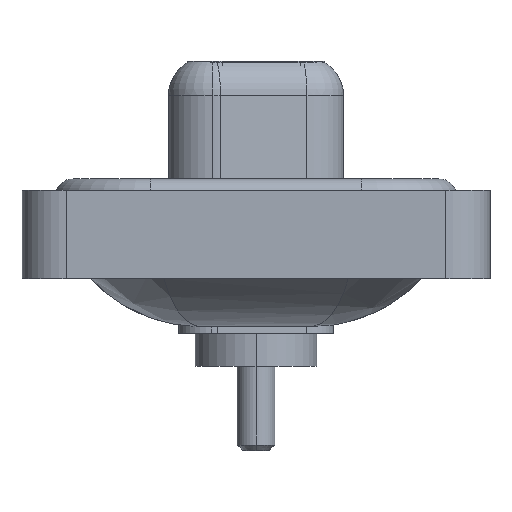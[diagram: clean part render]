
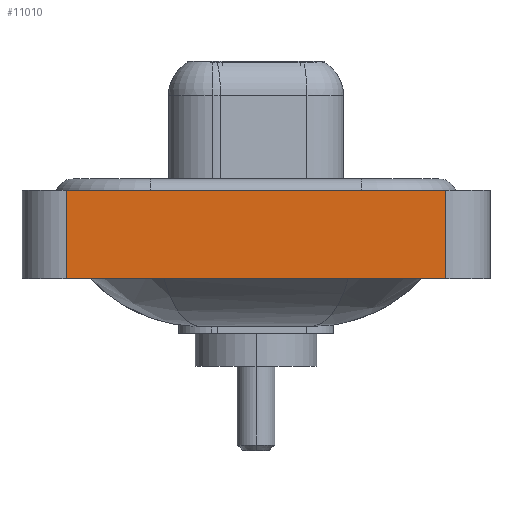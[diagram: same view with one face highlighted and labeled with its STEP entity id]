
A CAD part, left-side view. The second image highlights one B-rep face of the part: STEP entity #11010.
In plain terms, the highlighted planar face has unit normal (-1, 0, 0).
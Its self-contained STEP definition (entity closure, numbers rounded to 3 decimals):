
#503 = VERTEX_POINT ( 'NONE', #1447 ) ;
#768 = CARTESIAN_POINT ( 'NONE',  ( -7.25, 8.55, -3.6 ) ) ;
#1003 = VECTOR ( 'NONE', #8576, 1000. ) ;
#1018 = FACE_OUTER_BOUND ( 'NONE', #13302, .T. ) ;
#1052 = ORIENTED_EDGE ( 'NONE', *, *, #15396, .T. ) ;
#1237 = VECTOR ( 'NONE', #14821, 1000. ) ;
#1447 = CARTESIAN_POINT ( 'NONE',  ( -7.25, -8.55, 0.4 ) ) ;
#2682 = DIRECTION ( 'NONE',  ( -1., 0., 0. ) ) ;
#2829 = CARTESIAN_POINT ( 'NONE',  ( -7.25, -8.55, -3.6 ) ) ;
#3070 = CARTESIAN_POINT ( 'NONE',  ( -7.25, -8.55, 0.4 ) ) ;
#3627 = PLANE ( 'NONE',  #10861 ) ;
#4041 = VECTOR ( 'NONE', #7877, 1000. ) ;
#4417 = LINE ( 'NONE', #3070, #8654 ) ;
#5239 = VERTEX_POINT ( 'NONE', #16526 ) ;
#5352 = CARTESIAN_POINT ( 'NONE',  ( -7.25, 8.55, -3.6 ) ) ;
#5769 = EDGE_CURVE ( 'NONE', #6599, #503, #4417, .T. ) ;
#5808 = CARTESIAN_POINT ( 'NONE',  ( -7.25, -8.55, -3.6 ) ) ;
#5853 = ORIENTED_EDGE ( 'NONE', *, *, #12767, .F. ) ;
#6394 = DIRECTION ( 'NONE',  ( 0., 0., 1. ) ) ;
#6599 = VERTEX_POINT ( 'NONE', #8038 ) ;
#7877 = DIRECTION ( 'NONE',  ( 0., -1., 0. ) ) ;
#8038 = CARTESIAN_POINT ( 'NONE',  ( -7.25, 8.55, 0.4 ) ) ;
#8187 = DIRECTION ( 'NONE',  ( 0., -1., 0. ) ) ;
#8576 = DIRECTION ( 'NONE',  ( 0., 0., 1. ) ) ;
#8654 = VECTOR ( 'NONE', #8187, 1000. ) ;
#9137 = LINE ( 'NONE', #2829, #4041 ) ;
#9482 = ORIENTED_EDGE ( 'NONE', *, *, #5769, .F. ) ;
#10861 = AXIS2_PLACEMENT_3D ( 'NONE', #16518, #2682, #6394 ) ;
#11010 = ADVANCED_FACE ( 'NONE', ( #1018 ), #3627, .T. ) ;
#12087 = ORIENTED_EDGE ( 'NONE', *, *, #13985, .T. ) ;
#12767 = EDGE_CURVE ( 'NONE', #13062, #6599, #13229, .T. ) ;
#13062 = VERTEX_POINT ( 'NONE', #5352 ) ;
#13229 = LINE ( 'NONE', #768, #1237 ) ;
#13302 = EDGE_LOOP ( 'NONE', ( #12087, #9482, #5853, #1052 ) ) ;
#13985 = EDGE_CURVE ( 'NONE', #5239, #503, #15996, .T. ) ;
#14821 = DIRECTION ( 'NONE',  ( 0., 0., 1. ) ) ;
#15396 = EDGE_CURVE ( 'NONE', #13062, #5239, #9137, .T. ) ;
#15996 = LINE ( 'NONE', #5808, #1003 ) ;
#16518 = CARTESIAN_POINT ( 'NONE',  ( -7.25, -8.55, -3.6 ) ) ;
#16526 = CARTESIAN_POINT ( 'NONE',  ( -7.25, -8.55, -3.6 ) ) ;
